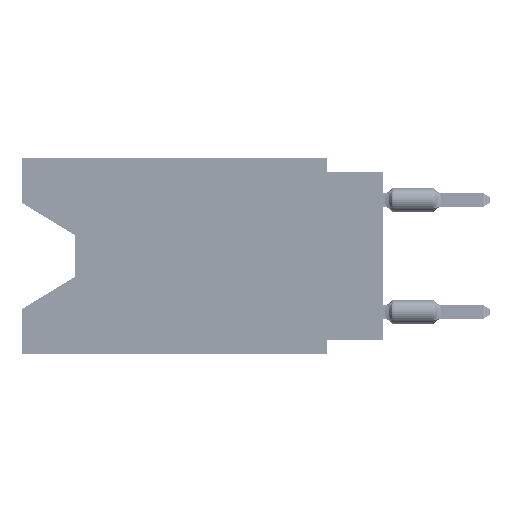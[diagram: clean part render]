
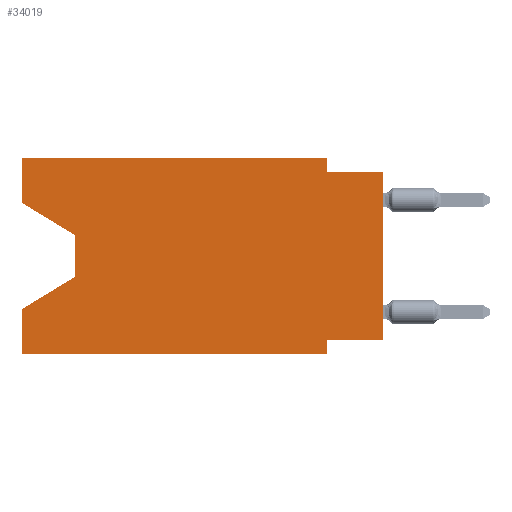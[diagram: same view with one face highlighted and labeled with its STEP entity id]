
A CAD part, left-side view. The second image highlights one B-rep face of the part: STEP entity #34019.
In plain terms, the highlighted planar face has unit normal (-1, 0, 0).
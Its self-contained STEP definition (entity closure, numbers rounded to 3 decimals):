
#914 = EDGE_CURVE ( 'NONE', #54916, #24253, #90286, .T. ) ;
#2124 = CARTESIAN_POINT ( 'NONE',  ( 0., 0., -0.635 ) ) ;
#2451 = DIRECTION ( 'NONE',  ( 0., -1., 0. ) ) ;
#3627 = CARTESIAN_POINT ( 'NONE',  ( 0., 16.383, -2.038 ) ) ;
#4203 = VERTEX_POINT ( 'NONE', #75650 ) ;
#6030 = EDGE_LOOP ( 'NONE', ( #86249, #76050, #89021, #16649, #23325, #25292, #33834, #12005, #86277, #76406, #71304, #85796 ) ) ;
#6216 = LINE ( 'NONE', #34730, #40304 ) ;
#7089 = CARTESIAN_POINT ( 'NONE',  ( 0., 13.97, -5.385 ) ) ;
#7847 = VERTEX_POINT ( 'NONE', #17063 ) ;
#8602 = EDGE_CURVE ( 'NONE', #54916, #9149, #64233, .T. ) ;
#8767 = LINE ( 'NONE', #38695, #52831 ) ;
#9149 = VERTEX_POINT ( 'NONE', #2124 ) ;
#9361 = VECTOR ( 'NONE', #14800, 1000. ) ;
#9683 = CARTESIAN_POINT ( 'NONE',  ( 0., 16.383, 0. ) ) ;
#10922 = LINE ( 'NONE', #20058, #83812 ) ;
#12005 = ORIENTED_EDGE ( 'NONE', *, *, #8602, .T. ) ;
#14800 = DIRECTION ( 'NONE',  ( 0., 0.855, -0.519 ) ) ;
#16649 = ORIENTED_EDGE ( 'NONE', *, *, #85455, .F. ) ;
#17063 = CARTESIAN_POINT ( 'NONE',  ( 0., 2.54, 0. ) ) ;
#18966 = CARTESIAN_POINT ( 'NONE',  ( 0., 16.383, 0. ) ) ;
#19287 = CARTESIAN_POINT ( 'NONE',  ( 0., 2.54, -8.89 ) ) ;
#19629 = VECTOR ( 'NONE', #87848, 1000. ) ;
#20058 = CARTESIAN_POINT ( 'NONE',  ( 0., 13.97, -3.505 ) ) ;
#20792 = CARTESIAN_POINT ( 'NONE',  ( 0., 2.54, 0. ) ) ;
#20839 = PLANE ( 'NONE',  #23050 ) ;
#23050 = AXIS2_PLACEMENT_3D ( 'NONE', #18966, #72064, #49843 ) ;
#23325 = ORIENTED_EDGE ( 'NONE', *, *, #34542, .T. ) ;
#24253 = VERTEX_POINT ( 'NONE', #79881 ) ;
#25292 = ORIENTED_EDGE ( 'NONE', *, *, #60426, .F. ) ;
#26774 = VECTOR ( 'NONE', #56966, 1000. ) ;
#26824 = EDGE_CURVE ( 'NONE', #50614, #87535, #27706, .T. ) ;
#27497 = CARTESIAN_POINT ( 'NONE',  ( 0., 0., 0. ) ) ;
#27706 = LINE ( 'NONE', #3627, #29855 ) ;
#27866 = EDGE_CURVE ( 'NONE', #35559, #7847, #83576, .T. ) ;
#29855 = VECTOR ( 'NONE', #41277, 1000. ) ;
#30898 = CARTESIAN_POINT ( 'NONE',  ( 0., 13.97, -3.505 ) ) ;
#32283 = DIRECTION ( 'NONE',  ( 0., 1., 0. ) ) ;
#33834 = ORIENTED_EDGE ( 'NONE', *, *, #914, .F. ) ;
#33869 = LINE ( 'NONE', #20792, #83214 ) ;
#34019 = ADVANCED_FACE ( 'NONE', ( #79301 ), #20839, .F. ) ;
#34542 = EDGE_CURVE ( 'NONE', #77813, #94620, #65169, .T. ) ;
#34730 = CARTESIAN_POINT ( 'NONE',  ( 0., 2.54, -8.89 ) ) ;
#34811 = EDGE_CURVE ( 'NONE', #4203, #35045, #94047, .T. ) ;
#35045 = VERTEX_POINT ( 'NONE', #83795 ) ;
#35559 = VERTEX_POINT ( 'NONE', #56588 ) ;
#38695 = CARTESIAN_POINT ( 'NONE',  ( 0., 16.383, 0. ) ) ;
#39550 = CARTESIAN_POINT ( 'NONE',  ( 0., 0., -8.255 ) ) ;
#39922 = EDGE_CURVE ( 'NONE', #7847, #45649, #33869, .T. ) ;
#40304 = VECTOR ( 'NONE', #64204, 1000. ) ;
#41277 = DIRECTION ( 'NONE',  ( 0., -0.855, -0.519 ) ) ;
#43924 = VECTOR ( 'NONE', #2451, 1000. ) ;
#45649 = VERTEX_POINT ( 'NONE', #76129 ) ;
#48854 = DIRECTION ( 'NONE',  ( 0., 0., -1. ) ) ;
#49843 = DIRECTION ( 'NONE',  ( 0., 0., -1. ) ) ;
#50614 = VERTEX_POINT ( 'NONE', #80575 ) ;
#52831 = VECTOR ( 'NONE', #61406, 1000. ) ;
#53674 = CARTESIAN_POINT ( 'NONE',  ( 0., 0., -8.255 ) ) ;
#54173 = VECTOR ( 'NONE', #82112, 1000. ) ;
#54226 = EDGE_CURVE ( 'NONE', #45649, #9149, #95095, .T. ) ;
#54916 = VERTEX_POINT ( 'NONE', #53674 ) ;
#56588 = CARTESIAN_POINT ( 'NONE',  ( 0., 16.383, 0. ) ) ;
#56966 = DIRECTION ( 'NONE',  ( 0., 0., 1. ) ) ;
#58258 = EDGE_CURVE ( 'NONE', #50614, #35559, #75334, .T. ) ;
#58380 = CARTESIAN_POINT ( 'NONE',  ( 0., 0., -0.635 ) ) ;
#60426 = EDGE_CURVE ( 'NONE', #24253, #94620, #6216, .T. ) ;
#61406 = DIRECTION ( 'NONE',  ( 0., 0., 1. ) ) ;
#64204 = DIRECTION ( 'NONE',  ( 0., 0., -1. ) ) ;
#64233 = LINE ( 'NONE', #27497, #26774 ) ;
#64561 = CARTESIAN_POINT ( 'NONE',  ( 0., 16.383, -8.89 ) ) ;
#65169 = LINE ( 'NONE', #94639, #72510 ) ;
#65645 = DIRECTION ( 'NONE',  ( 0., -1., 0. ) ) ;
#71304 = ORIENTED_EDGE ( 'NONE', *, *, #27866, .F. ) ;
#72064 = DIRECTION ( 'NONE',  ( 1., 0., 0. ) ) ;
#72510 = VECTOR ( 'NONE', #65645, 1000. ) ;
#75334 = LINE ( 'NONE', #88876, #54173 ) ;
#75650 = CARTESIAN_POINT ( 'NONE',  ( 0., 13.97, -5.385 ) ) ;
#76050 = ORIENTED_EDGE ( 'NONE', *, *, #86528, .T. ) ;
#76129 = CARTESIAN_POINT ( 'NONE',  ( 0., 2.54, -0.635 ) ) ;
#76406 = ORIENTED_EDGE ( 'NONE', *, *, #39922, .F. ) ;
#77813 = VERTEX_POINT ( 'NONE', #64561 ) ;
#79301 = FACE_OUTER_BOUND ( 'NONE', #6030, .T. ) ;
#79881 = CARTESIAN_POINT ( 'NONE',  ( 0., 2.54, -8.255 ) ) ;
#80575 = CARTESIAN_POINT ( 'NONE',  ( 0., 16.383, -2.038 ) ) ;
#82112 = DIRECTION ( 'NONE',  ( 0., 0., 1. ) ) ;
#83214 = VECTOR ( 'NONE', #48854, 1000. ) ;
#83576 = LINE ( 'NONE', #9683, #43924 ) ;
#83795 = CARTESIAN_POINT ( 'NONE',  ( 0., 16.383, -6.852 ) ) ;
#83812 = VECTOR ( 'NONE', #94921, 1000. ) ;
#85455 = EDGE_CURVE ( 'NONE', #77813, #35045, #8767, .T. ) ;
#85796 = ORIENTED_EDGE ( 'NONE', *, *, #58258, .F. ) ;
#86249 = ORIENTED_EDGE ( 'NONE', *, *, #26824, .T. ) ;
#86277 = ORIENTED_EDGE ( 'NONE', *, *, #54226, .F. ) ;
#86528 = EDGE_CURVE ( 'NONE', #87535, #4203, #10922, .T. ) ;
#87535 = VERTEX_POINT ( 'NONE', #30898 ) ;
#87848 = DIRECTION ( 'NONE',  ( 0., -1., 0. ) ) ;
#88876 = CARTESIAN_POINT ( 'NONE',  ( 0., 16.383, 0. ) ) ;
#89021 = ORIENTED_EDGE ( 'NONE', *, *, #34811, .T. ) ;
#90286 = LINE ( 'NONE', #39550, #95168 ) ;
#94047 = LINE ( 'NONE', #7089, #9361 ) ;
#94620 = VERTEX_POINT ( 'NONE', #19287 ) ;
#94639 = CARTESIAN_POINT ( 'NONE',  ( 0., 16.383, -8.89 ) ) ;
#94921 = DIRECTION ( 'NONE',  ( 0., 0., -1. ) ) ;
#95095 = LINE ( 'NONE', #58380, #19629 ) ;
#95168 = VECTOR ( 'NONE', #32283, 1000. ) ;
